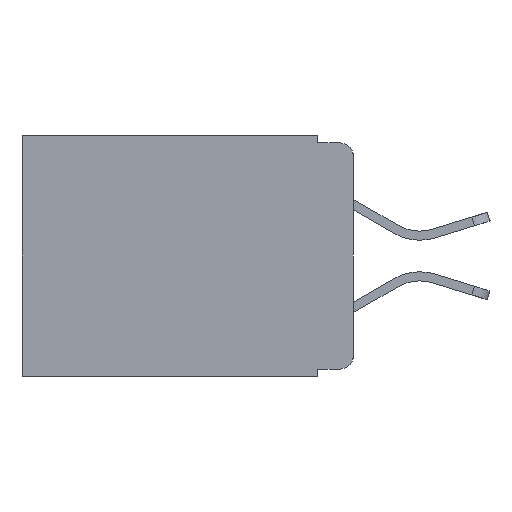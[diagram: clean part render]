
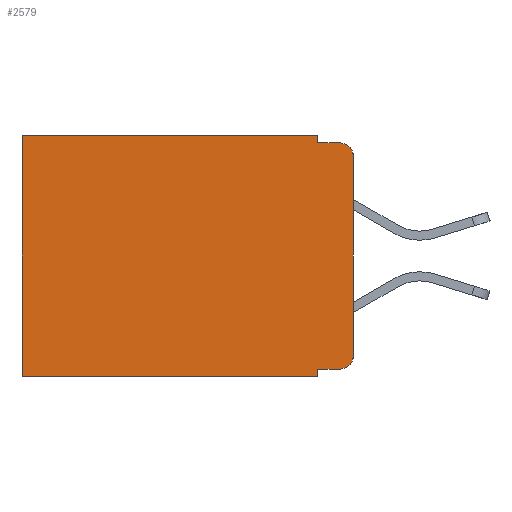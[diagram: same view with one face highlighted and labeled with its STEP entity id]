
A CAD part, left-side view. The second image highlights one B-rep face of the part: STEP entity #2579.
In plain terms, the highlighted planar face has unit normal (-1, 0, 0).
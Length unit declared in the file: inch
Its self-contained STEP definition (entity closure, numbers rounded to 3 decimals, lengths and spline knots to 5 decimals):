
#258 = LINE ( 'NONE', #1695, #16792 ) ;
#479 = DIRECTION ( 'NONE',  ( 0., 1., 0. ) ) ;
#829 = LINE ( 'NONE', #2919, #8452 ) ;
#1027 = EDGE_CURVE ( 'NONE', #20035, #9567, #12146, .T. ) ;
#1501 = CARTESIAN_POINT ( 'NONE',  ( 0.298, 0.02, -0.313 ) ) ;
#1628 = LINE ( 'NONE', #16411, #13822 ) ;
#1695 = CARTESIAN_POINT ( 'NONE',  ( 0.298, 0., 0. ) ) ;
#1951 = VECTOR ( 'NONE', #10738, 39.37008 ) ;
#2579 = ADVANCED_FACE ( 'NONE', ( #18293 ), #13147, .F. ) ;
#2592 = EDGE_LOOP ( 'NONE', ( #9506, #11759, #14696, #3170, #3361, #3529, #4958, #5145, #9555, #10864 ) ) ;
#2834 = CIRCLE ( 'NONE', #7965, 0.02 ) ;
#2919 = CARTESIAN_POINT ( 'NONE',  ( 0.298, 0.051, -0.333 ) ) ;
#3114 = EDGE_CURVE ( 'NONE', #4583, #14110, #258, .T. ) ;
#3170 = ORIENTED_EDGE ( 'NONE', *, *, #10561, .F. ) ;
#3204 = DIRECTION ( 'NONE',  ( 0., 0., -1. ) ) ;
#3224 = CARTESIAN_POINT ( 'NONE',  ( 0.298, 0.473, 0. ) ) ;
#3361 = ORIENTED_EDGE ( 'NONE', *, *, #1027, .T. ) ;
#3483 = CIRCLE ( 'NONE', #7652, 0.02 ) ;
#3529 = ORIENTED_EDGE ( 'NONE', *, *, #11603, .T. ) ;
#3739 = CARTESIAN_POINT ( 'NONE',  ( 0.298, 0., 0. ) ) ;
#3753 = CARTESIAN_POINT ( 'NONE',  ( 0.298, 0., 0. ) ) ;
#4583 = VERTEX_POINT ( 'NONE', #18182 ) ;
#4879 = LINE ( 'NONE', #18018, #20631 ) ;
#4958 = ORIENTED_EDGE ( 'NONE', *, *, #13453, .F. ) ;
#5145 = ORIENTED_EDGE ( 'NONE', *, *, #14791, .F. ) ;
#5345 = DIRECTION ( 'NONE',  ( 0., 0., -1. ) ) ;
#5694 = CARTESIAN_POINT ( 'NONE',  ( 0.298, 0.02, -0.333 ) ) ;
#6045 = CARTESIAN_POINT ( 'NONE',  ( 0.298, 0.051, 0. ) ) ;
#6377 = CARTESIAN_POINT ( 'NONE',  ( 0.298, 0., -0.313 ) ) ;
#6594 = VERTEX_POINT ( 'NONE', #15460 ) ;
#7370 = EDGE_CURVE ( 'NONE', #4583, #8565, #3483, .T. ) ;
#7652 = AXIS2_PLACEMENT_3D ( 'NONE', #17746, #8299, #19286 ) ;
#7965 = AXIS2_PLACEMENT_3D ( 'NONE', #1501, #12698, #3204 ) ;
#8165 = DIRECTION ( 'NONE',  ( 0., 0., -1. ) ) ;
#8299 = DIRECTION ( 'NONE',  ( -1., 0., 0. ) ) ;
#8452 = VECTOR ( 'NONE', #12427, 39.37008 ) ;
#8468 = EDGE_CURVE ( 'NONE', #6594, #8565, #16040, .T. ) ;
#8471 = CARTESIAN_POINT ( 'NONE',  ( 0.298, 0.051, -0.343 ) ) ;
#8565 = VERTEX_POINT ( 'NONE', #11767 ) ;
#8679 = VERTEX_POINT ( 'NONE', #5694 ) ;
#9099 = VERTEX_POINT ( 'NONE', #16218 ) ;
#9122 = CARTESIAN_POINT ( 'NONE',  ( 0.298, 0.051, -0.333 ) ) ;
#9506 = ORIENTED_EDGE ( 'NONE', *, *, #3114, .F. ) ;
#9555 = ORIENTED_EDGE ( 'NONE', *, *, #16906, .T. ) ;
#9567 = VERTEX_POINT ( 'NONE', #3224 ) ;
#10561 = EDGE_CURVE ( 'NONE', #20035, #6594, #19304, .T. ) ;
#10738 = DIRECTION ( 'NONE',  ( 0., 0., -1. ) ) ;
#10864 = ORIENTED_EDGE ( 'NONE', *, *, #20021, .T. ) ;
#10907 = VERTEX_POINT ( 'NONE', #8471 ) ;
#11499 = CARTESIAN_POINT ( 'NONE',  ( 0.298, 0.051, -0.01 ) ) ;
#11561 = DIRECTION ( 'NONE',  ( 0., -1., 0. ) ) ;
#11603 = EDGE_CURVE ( 'NONE', #9567, #9099, #1628, .T. ) ;
#11759 = ORIENTED_EDGE ( 'NONE', *, *, #7370, .T. ) ;
#11767 = CARTESIAN_POINT ( 'NONE',  ( 0.298, 0.02, -0.01 ) ) ;
#11850 = VECTOR ( 'NONE', #11561, 39.37008 ) ;
#12146 = LINE ( 'NONE', #3739, #20491 ) ;
#12427 = DIRECTION ( 'NONE',  ( 0., -1., 0. ) ) ;
#12698 = DIRECTION ( 'NONE',  ( -1., 0., 0. ) ) ;
#12775 = CARTESIAN_POINT ( 'NONE',  ( 0.298, 0.051, 0. ) ) ;
#13147 = PLANE ( 'NONE',  #18187 ) ;
#13453 = EDGE_CURVE ( 'NONE', #10907, #9099, #4879, .T. ) ;
#13822 = VECTOR ( 'NONE', #18015, 39.37008 ) ;
#14110 = VERTEX_POINT ( 'NONE', #6377 ) ;
#14326 = DIRECTION ( 'NONE',  ( 0., 0., -1. ) ) ;
#14696 = ORIENTED_EDGE ( 'NONE', *, *, #8468, .F. ) ;
#14791 = EDGE_CURVE ( 'NONE', #16813, #10907, #20564, .T. ) ;
#14801 = DIRECTION ( 'NONE',  ( 1., 0., 0. ) ) ;
#15460 = CARTESIAN_POINT ( 'NONE',  ( 0.298, 0.051, -0.01 ) ) ;
#16040 = LINE ( 'NONE', #11499, #11850 ) ;
#16218 = CARTESIAN_POINT ( 'NONE',  ( 0.298, 0.473, -0.343 ) ) ;
#16411 = CARTESIAN_POINT ( 'NONE',  ( 0.298, 0.473, 0. ) ) ;
#16780 = DIRECTION ( 'NONE',  ( 0., 1., 0. ) ) ;
#16792 = VECTOR ( 'NONE', #8165, 39.37008 ) ;
#16813 = VERTEX_POINT ( 'NONE', #9122 ) ;
#16906 = EDGE_CURVE ( 'NONE', #16813, #8679, #829, .T. ) ;
#17746 = CARTESIAN_POINT ( 'NONE',  ( 0.298, 0.02, -0.03 ) ) ;
#18015 = DIRECTION ( 'NONE',  ( 0., 0., -1. ) ) ;
#18018 = CARTESIAN_POINT ( 'NONE',  ( 0.298, 0., -0.343 ) ) ;
#18182 = CARTESIAN_POINT ( 'NONE',  ( 0.298, 0., -0.03 ) ) ;
#18187 = AXIS2_PLACEMENT_3D ( 'NONE', #3753, #14801, #5345 ) ;
#18293 = FACE_OUTER_BOUND ( 'NONE', #2592, .T. ) ;
#18942 = CARTESIAN_POINT ( 'NONE',  ( 0.298, 0.051, 0. ) ) ;
#19286 = DIRECTION ( 'NONE',  ( 0., 0., -1. ) ) ;
#19304 = LINE ( 'NONE', #6045, #1951 ) ;
#20021 = EDGE_CURVE ( 'NONE', #8679, #14110, #2834, .T. ) ;
#20035 = VERTEX_POINT ( 'NONE', #18942 ) ;
#20068 = VECTOR ( 'NONE', #14326, 39.37008 ) ;
#20491 = VECTOR ( 'NONE', #16780, 39.37008 ) ;
#20564 = LINE ( 'NONE', #12775, #20068 ) ;
#20631 = VECTOR ( 'NONE', #479, 39.37008 ) ;
